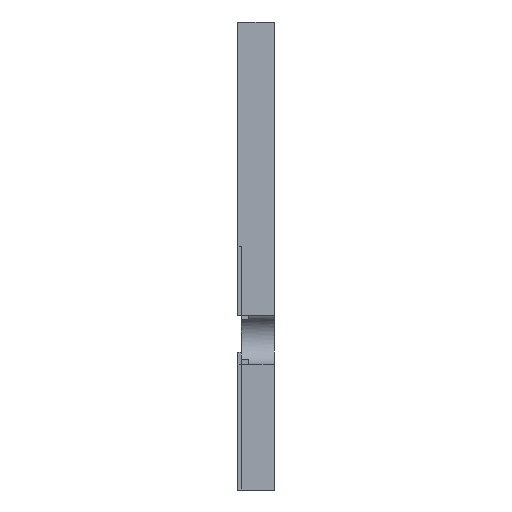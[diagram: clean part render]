
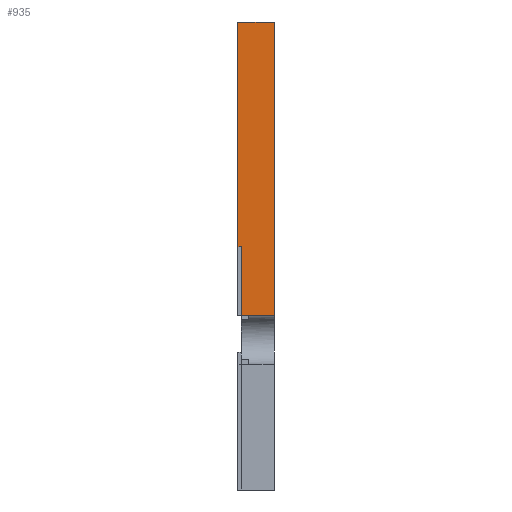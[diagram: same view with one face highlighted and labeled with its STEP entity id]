
A CAD part, left-side view. The second image highlights one B-rep face of the part: STEP entity #935.
In plain terms, the highlighted planar face has unit normal (-1, 0, 0).
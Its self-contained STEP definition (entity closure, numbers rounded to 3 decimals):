
#41 = DIRECTION ( 'NONE',  ( 0., 0., -1. ) ) ;
#51 = CARTESIAN_POINT ( 'NONE',  ( 0., -5., 0. ) ) ;
#71 = EDGE_CURVE ( 'NONE', #1266, #773, #251, .T. ) ;
#84 = CARTESIAN_POINT ( 'NONE',  ( 0., -5., -40.361 ) ) ;
#85 = CARTESIAN_POINT ( 'NONE',  ( 0., 0., 0. ) ) ;
#91 = ORIENTED_EDGE ( 'NONE', *, *, #257, .F. ) ;
#98 = DIRECTION ( 'NONE',  ( 0., 0., -1. ) ) ;
#127 = VECTOR ( 'NONE', #781, 1000. ) ;
#162 = CARTESIAN_POINT ( 'NONE',  ( 0., 0., 0. ) ) ;
#168 = CARTESIAN_POINT ( 'NONE',  ( 0., -5., 0. ) ) ;
#177 = CARTESIAN_POINT ( 'NONE',  ( 0., -5., -40.361 ) ) ;
#196 = CARTESIAN_POINT ( 'NONE',  ( 0., 0., -30.931 ) ) ;
#223 = EDGE_CURVE ( 'NONE', #813, #805, #455, .T. ) ;
#251 = LINE ( 'NONE', #1246, #1441 ) ;
#257 = EDGE_CURVE ( 'NONE', #377, #883, #758, .T. ) ;
#265 = DIRECTION ( 'NONE',  ( 0., 1., 0. ) ) ;
#312 = LINE ( 'NONE', #168, #1454 ) ;
#361 = CARTESIAN_POINT ( 'NONE',  ( 0., -0.533, -30.931 ) ) ;
#377 = VERTEX_POINT ( 'NONE', #177 ) ;
#441 = EDGE_CURVE ( 'NONE', #883, #1266, #1034, .T. ) ;
#455 = LINE ( 'NONE', #1358, #127 ) ;
#509 = ORIENTED_EDGE ( 'NONE', *, *, #814, .T. ) ;
#599 = FACE_OUTER_BOUND ( 'NONE', #1336, .T. ) ;
#636 = ORIENTED_EDGE ( 'NONE', *, *, #795, .F. ) ;
#733 = VECTOR ( 'NONE', #1375, 1000. ) ;
#758 = LINE ( 'NONE', #84, #1251 ) ;
#773 = VERTEX_POINT ( 'NONE', #196 ) ;
#781 = DIRECTION ( 'NONE',  ( 0., 1., 0. ) ) ;
#795 = EDGE_CURVE ( 'NONE', #813, #377, #312, .T. ) ;
#805 = VERTEX_POINT ( 'NONE', #162 ) ;
#813 = VERTEX_POINT ( 'NONE', #51 ) ;
#814 = EDGE_CURVE ( 'NONE', #805, #773, #876, .T. ) ;
#848 = CARTESIAN_POINT ( 'NONE',  ( 0., -0.533, -40.361 ) ) ;
#876 = LINE ( 'NONE', #85, #1420 ) ;
#883 = VERTEX_POINT ( 'NONE', #848 ) ;
#902 = DIRECTION ( 'NONE',  ( 0., 1., 0. ) ) ;
#935 = ADVANCED_FACE ( 'NONE', ( #599 ), #1064, .F. ) ;
#1002 = CARTESIAN_POINT ( 'NONE',  ( 0., -0.533, -30.931 ) ) ;
#1030 = DIRECTION ( 'NONE',  ( 0., 0., -1. ) ) ;
#1034 = LINE ( 'NONE', #361, #733 ) ;
#1059 = CARTESIAN_POINT ( 'NONE',  ( 0., -5., 0. ) ) ;
#1064 = PLANE ( 'NONE',  #1369 ) ;
#1160 = DIRECTION ( 'NONE',  ( 1., 0., 0. ) ) ;
#1206 = ORIENTED_EDGE ( 'NONE', *, *, #71, .F. ) ;
#1246 = CARTESIAN_POINT ( 'NONE',  ( 0., -0.533, -30.931 ) ) ;
#1251 = VECTOR ( 'NONE', #902, 1000. ) ;
#1266 = VERTEX_POINT ( 'NONE', #1002 ) ;
#1315 = ORIENTED_EDGE ( 'NONE', *, *, #223, .T. ) ;
#1336 = EDGE_LOOP ( 'NONE', ( #509, #1206, #1445, #91, #636, #1315 ) ) ;
#1358 = CARTESIAN_POINT ( 'NONE',  ( 0., -5., 0. ) ) ;
#1369 = AXIS2_PLACEMENT_3D ( 'NONE', #1059, #1160, #1030 ) ;
#1375 = DIRECTION ( 'NONE',  ( 0., 0., 1. ) ) ;
#1420 = VECTOR ( 'NONE', #41, 1000. ) ;
#1441 = VECTOR ( 'NONE', #265, 1000. ) ;
#1445 = ORIENTED_EDGE ( 'NONE', *, *, #441, .F. ) ;
#1454 = VECTOR ( 'NONE', #98, 1000. ) ;
